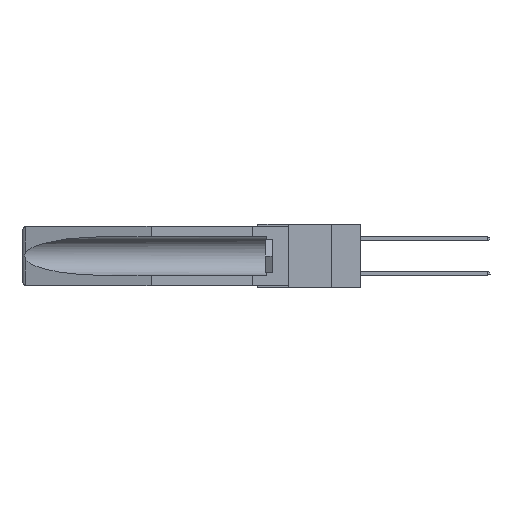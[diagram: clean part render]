
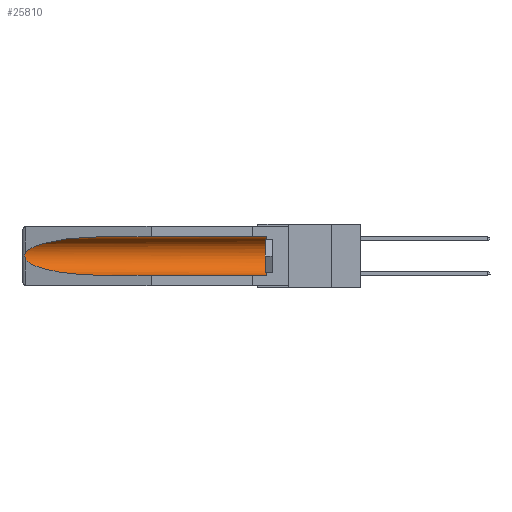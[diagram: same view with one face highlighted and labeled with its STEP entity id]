
A CAD part, left-side view. The second image highlights one B-rep face of the part: STEP entity #25810.
In plain terms, the highlighted cylindrical face has radius 2.857 mm (diameter 5.715 mm), a partial arc.
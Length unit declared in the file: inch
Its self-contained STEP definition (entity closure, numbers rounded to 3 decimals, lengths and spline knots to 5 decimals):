
#833 = CARTESIAN_POINT ( 'NONE',  ( 0.2675, 1.53308, -0.17534 ) ) ;
#918 = CARTESIAN_POINT ( 'NONE',  ( 0.2673, 1.5327, -0.16383 ) ) ;
#1375 = LINE ( 'NONE', #10438, #27038 ) ;
#1411 = DIRECTION ( 'NONE',  ( 0., 0., 1. ) ) ;
#1957 = ORIENTED_EDGE ( 'NONE', *, *, #7077, .T. ) ;
#2009 = ORIENTED_EDGE ( 'NONE', *, *, #18960, .T. ) ;
#2149 = FACE_OUTER_BOUND ( 'NONE', #8458, .T. ) ;
#2337 = VECTOR ( 'NONE', #24919, 39.37008 ) ;
#2581 = VERTEX_POINT ( 'NONE', #3878 ) ;
#3013 = CARTESIAN_POINT ( 'NONE',  ( 0.26655, 1.53094, -0.18657 ) ) ;
#3491 = CARTESIAN_POINT ( 'NONE',  ( 0.155, 0.126, -0.1715 ) ) ;
#3878 = CARTESIAN_POINT ( 'NONE',  ( 0.26537, 1.52718, -0.19328 ) ) ;
#4259 = DIRECTION ( 'NONE',  ( 0., 1., 0. ) ) ;
#4448 = CARTESIAN_POINT ( 'NONE',  ( 0.155, 1.07973, -0.284 ) ) ;
#5086 =( BOUNDED_CURVE ( )  B_SPLINE_CURVE ( 3, ( #17904, #26221, #17820, #5153 ),
 .UNSPECIFIED., .F., .F. ) 
 B_SPLINE_CURVE_WITH_KNOTS ( ( 4, 4 ),
 ( 4.71239, 6.08839 ),
 .UNSPECIFIED. ) 
 CURVE ( )  GEOMETRIC_REPRESENTATION_ITEM ( )  RATIONAL_B_SPLINE_CURVE ( ( 1., 0.848, 0.848, 1. ) ) 
 REPRESENTATION_ITEM ( '' )  );
#5153 = CARTESIAN_POINT ( 'NONE',  ( 0.26537, 1.52718, -0.14972 ) ) ;
#5286 = ORIENTED_EDGE ( 'NONE', *, *, #24789, .T. ) ;
#6403 = EDGE_CURVE ( 'NONE', #6484, #18928, #1375, .T. ) ;
#6411 = CYLINDRICAL_SURFACE ( 'NONE', #16884, 0.1125 ) ;
#6441 = CARTESIAN_POINT ( 'NONE',  ( 0.155, -0.30754, -0.1715 ) ) ;
#6484 = VERTEX_POINT ( 'NONE', #16184 ) ;
#7077 = EDGE_CURVE ( 'NONE', #10872, #8110, #5086, .T. ) ;
#7099 = CARTESIAN_POINT ( 'NONE',  ( 0.155, 1.07973, -0.059 ) ) ;
#7389 = CARTESIAN_POINT ( 'NONE',  ( 0.25451, 1.48313, -0.24835 ) ) ;
#7877 = VERTEX_POINT ( 'NONE', #12723 ) ;
#8110 = VERTEX_POINT ( 'NONE', #18668 ) ;
#8458 = EDGE_LOOP ( 'NONE', ( #1957, #19278, #2009, #24014, #5286, #11090 ) ) ;
#9180 = CARTESIAN_POINT ( 'NONE',  ( 0.26537, 1.52718, -0.14972 ) ) ;
#9888 = LINE ( 'NONE', #20951, #2337 ) ;
#10438 = CARTESIAN_POINT ( 'NONE',  ( 0.155, -0.30754, -0.284 ) ) ;
#10666 = DIRECTION ( 'NONE',  ( 0., 1., 0. ) ) ;
#10872 = VERTEX_POINT ( 'NONE', #7099 ) ;
#11090 = ORIENTED_EDGE ( 'NONE', *, *, #21857, .T. ) ;
#11284 = CARTESIAN_POINT ( 'NONE',  ( 0.2675, 1.53308, -0.16763 ) ) ;
#11814 = CARTESIAN_POINT ( 'NONE',  ( 0.21114, 1.30732, -0.284 ) ) ;
#12723 = CARTESIAN_POINT ( 'NONE',  ( 0.155, 0.126, -0.059 ) ) ;
#15375 = CIRCLE ( 'NONE', #25436, 0.1125 ) ;
#15647 = CARTESIAN_POINT ( 'NONE',  ( 0.2673, 1.53269, -0.17917 ) ) ;
#16184 = CARTESIAN_POINT ( 'NONE',  ( 0.155, 0.126, -0.284 ) ) ;
#16884 = AXIS2_PLACEMENT_3D ( 'NONE', #6441, #10666, #19157 ) ;
#17463 = B_SPLINE_CURVE_WITH_KNOTS ( 'NONE', 3,
 ( #9180, #23887, #19961, #918, #11284, #833, #15647, #3013, #17693, #19780 ),
 .UNSPECIFIED., .F., .F.,
 ( 4, 2, 2, 2, 4 ),
 ( 0., 0.00029, 0.00058, 0.00087, 0.00117 ),
 .UNSPECIFIED. ) ;
#17693 = CARTESIAN_POINT ( 'NONE',  ( 0.26597, 1.5296, -0.19026 ) ) ;
#17820 = CARTESIAN_POINT ( 'NONE',  ( 0.25451, 1.48313, -0.09465 ) ) ;
#17904 = CARTESIAN_POINT ( 'NONE',  ( 0.155, 1.07973, -0.059 ) ) ;
#18668 = CARTESIAN_POINT ( 'NONE',  ( 0.26537, 1.52718, -0.14972 ) ) ;
#18928 = VERTEX_POINT ( 'NONE', #4448 ) ;
#18960 = EDGE_CURVE ( 'NONE', #2581, #18928, #23125, .T. ) ;
#19157 = DIRECTION ( 'NONE',  ( 0., 0., 1. ) ) ;
#19278 = ORIENTED_EDGE ( 'NONE', *, *, #20714, .T. ) ;
#19780 = CARTESIAN_POINT ( 'NONE',  ( 0.26537, 1.52718, -0.19328 ) ) ;
#19961 = CARTESIAN_POINT ( 'NONE',  ( 0.26654, 1.53092, -0.15636 ) ) ;
#20194 = DIRECTION ( 'NONE',  ( 0., -1., 0. ) ) ;
#20714 = EDGE_CURVE ( 'NONE', #8110, #2581, #17463, .T. ) ;
#20951 = CARTESIAN_POINT ( 'NONE',  ( 0.155, -0.30754, -0.059 ) ) ;
#21857 = EDGE_CURVE ( 'NONE', #7877, #10872, #9888, .T. ) ;
#23125 =( BOUNDED_CURVE ( )  B_SPLINE_CURVE ( 3, ( #24397, #7389, #11814, #26349 ),
 .UNSPECIFIED., .F., .F. ) 
 B_SPLINE_CURVE_WITH_KNOTS ( ( 4, 4 ),
 ( 0.1948, 1.5708 ),
 .UNSPECIFIED. ) 
 CURVE ( )  GEOMETRIC_REPRESENTATION_ITEM ( )  RATIONAL_B_SPLINE_CURVE ( ( 1., 0.848, 0.848, 1. ) ) 
 REPRESENTATION_ITEM ( '' )  );
#23887 = CARTESIAN_POINT ( 'NONE',  ( 0.26597, 1.52961, -0.15275 ) ) ;
#24014 = ORIENTED_EDGE ( 'NONE', *, *, #6403, .F. ) ;
#24397 = CARTESIAN_POINT ( 'NONE',  ( 0.26537, 1.52718, -0.19328 ) ) ;
#24789 = EDGE_CURVE ( 'NONE', #6484, #7877, #15375, .T. ) ;
#24919 = DIRECTION ( 'NONE',  ( 0., 1., 0. ) ) ;
#25436 = AXIS2_PLACEMENT_3D ( 'NONE', #3491, #20194, #1411 ) ;
#25810 = ADVANCED_FACE ( 'NONE', ( #2149 ), #6411, .F. ) ;
#26221 = CARTESIAN_POINT ( 'NONE',  ( 0.21114, 1.30732, -0.059 ) ) ;
#26349 = CARTESIAN_POINT ( 'NONE',  ( 0.155, 1.07973, -0.284 ) ) ;
#27038 = VECTOR ( 'NONE', #4259, 39.37008 ) ;
